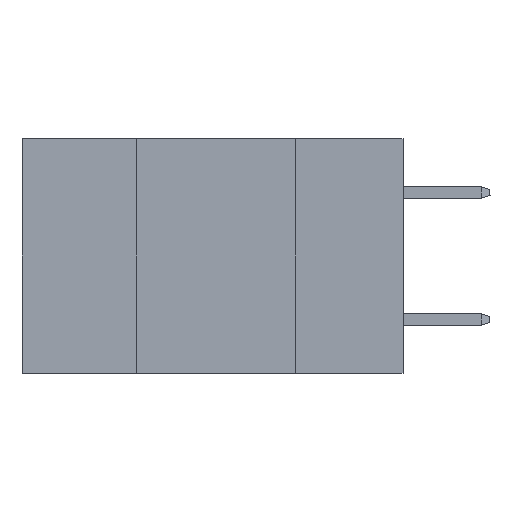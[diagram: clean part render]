
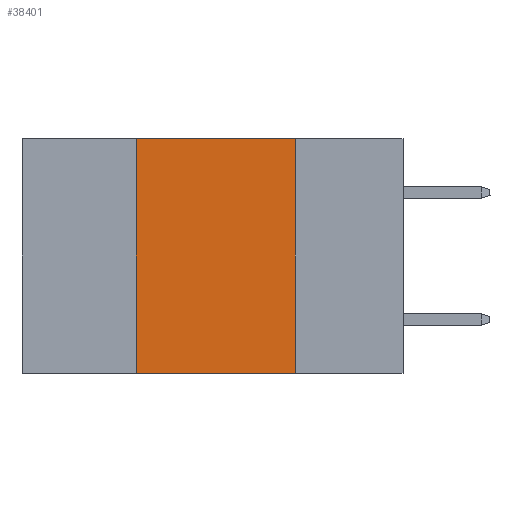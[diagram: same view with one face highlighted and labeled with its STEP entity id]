
A CAD part, left-side view. The second image highlights one B-rep face of the part: STEP entity #38401.
In plain terms, the highlighted planar face has unit normal (-1, 0, 0).
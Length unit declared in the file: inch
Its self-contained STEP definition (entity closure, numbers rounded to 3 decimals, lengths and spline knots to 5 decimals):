
#365 = EDGE_CURVE ( 'NONE', #1046, #23158, #25591, .T. ) ;
#395 = DIRECTION ( 'NONE',  ( 0., 0., -1. ) ) ;
#865 = CARTESIAN_POINT ( 'NONE',  ( 0., 0.6, 0. ) ) ;
#947 = CARTESIAN_POINT ( 'NONE',  ( 0., 0.17, 0. ) ) ;
#994 = PLANE ( 'NONE',  #39199 ) ;
#1046 = VERTEX_POINT ( 'NONE', #20457 ) ;
#1777 = EDGE_CURVE ( 'NONE', #20966, #28191, #31639, .T. ) ;
#2630 = ORIENTED_EDGE ( 'NONE', *, *, #23553, .F. ) ;
#4356 = LINE ( 'NONE', #947, #10117 ) ;
#6328 = LINE ( 'NONE', #33866, #26712 ) ;
#6785 = DIRECTION ( 'NONE',  ( 0., 0., -1. ) ) ;
#7660 = VECTOR ( 'NONE', #16736, 39.37008 ) ;
#8234 = CARTESIAN_POINT ( 'NONE',  ( 0., 0.42, -0.37 ) ) ;
#8898 = DIRECTION ( 'NONE',  ( 1., 0., 0. ) ) ;
#10117 = VECTOR ( 'NONE', #6785, 39.37008 ) ;
#12367 = ORIENTED_EDGE ( 'NONE', *, *, #1777, .T. ) ;
#15887 = VECTOR ( 'NONE', #28194, 39.37008 ) ;
#16736 = DIRECTION ( 'NONE',  ( 0., -1., 0. ) ) ;
#18015 = ORIENTED_EDGE ( 'NONE', *, *, #35420, .F. ) ;
#20050 = CARTESIAN_POINT ( 'NONE',  ( 0., 0.17, 0. ) ) ;
#20457 = CARTESIAN_POINT ( 'NONE',  ( 0., 0.42, 0. ) ) ;
#20966 = VERTEX_POINT ( 'NONE', #8234 ) ;
#21106 = ORIENTED_EDGE ( 'NONE', *, *, #365, .F. ) ;
#22121 = FACE_OUTER_BOUND ( 'NONE', #38615, .T. ) ;
#23158 = VERTEX_POINT ( 'NONE', #20050 ) ;
#23553 = EDGE_CURVE ( 'NONE', #20966, #1046, #6328, .T. ) ;
#24918 = CARTESIAN_POINT ( 'NONE',  ( 0., 0.6, 0. ) ) ;
#25535 = CARTESIAN_POINT ( 'NONE',  ( 0., 0.17, -0.37 ) ) ;
#25591 = LINE ( 'NONE', #865, #15887 ) ;
#26712 = VECTOR ( 'NONE', #30850, 39.37008 ) ;
#28191 = VERTEX_POINT ( 'NONE', #25535 ) ;
#28194 = DIRECTION ( 'NONE',  ( 0., -1., 0. ) ) ;
#30850 = DIRECTION ( 'NONE',  ( 0., 0., 1. ) ) ;
#31639 = LINE ( 'NONE', #34243, #7660 ) ;
#33866 = CARTESIAN_POINT ( 'NONE',  ( 0., 0.42, 0. ) ) ;
#34243 = CARTESIAN_POINT ( 'NONE',  ( 0., 0.6, -0.37 ) ) ;
#35420 = EDGE_CURVE ( 'NONE', #23158, #28191, #4356, .T. ) ;
#38401 = ADVANCED_FACE ( 'NONE', ( #22121 ), #994, .F. ) ;
#38615 = EDGE_LOOP ( 'NONE', ( #18015, #21106, #2630, #12367 ) ) ;
#39199 = AXIS2_PLACEMENT_3D ( 'NONE', #24918, #8898, #395 ) ;
